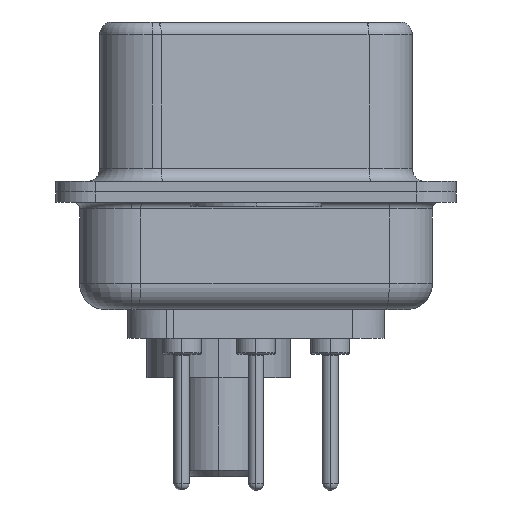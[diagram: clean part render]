
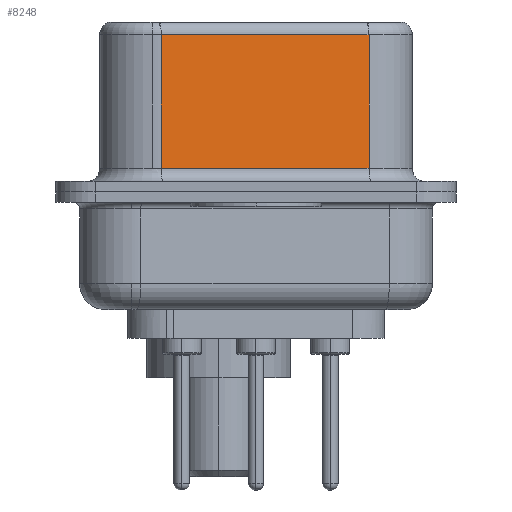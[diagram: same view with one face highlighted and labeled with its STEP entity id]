
A CAD part, left-side view. The second image highlights one B-rep face of the part: STEP entity #8248.
In plain terms, the highlighted planar face has unit normal (-0.985, -0.174, 0).
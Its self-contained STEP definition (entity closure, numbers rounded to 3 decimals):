
#238 = DIRECTION ( 'NONE',  ( 0.985, 0.174, 0. ) ) ;
#2399 = ORIENTED_EDGE ( 'NONE', *, *, #17463, .T. ) ;
#2860 = LINE ( 'NONE', #15412, #23816 ) ;
#3398 = CARTESIAN_POINT ( 'NONE',  ( 5.132, -4.322, 0.9 ) ) ;
#4527 = VERTEX_POINT ( 'NONE', #22207 ) ;
#5184 = VECTOR ( 'NONE', #6916, 1000. ) ;
#6916 = DIRECTION ( 'NONE',  ( 0., 0., -1. ) ) ;
#8248 = ADVANCED_FACE ( 'NONE', ( #8798 ), #12422, .F. ) ;
#8433 = CARTESIAN_POINT ( 'NONE',  ( 5.132, -4.322, 6.52 ) ) ;
#8798 = FACE_OUTER_BOUND ( 'NONE', #22012, .T. ) ;
#9192 = LINE ( 'NONE', #12974, #25461 ) ;
#9253 = VERTEX_POINT ( 'NONE', #9513 ) ;
#9513 = CARTESIAN_POINT ( 'NONE',  ( 3.73, 3.628, 0.9 ) ) ;
#10468 = LINE ( 'NONE', #14856, #5184 ) ;
#12422 = PLANE ( 'NONE',  #13414 ) ;
#12682 = VECTOR ( 'NONE', #23684, 1000. ) ;
#12974 = CARTESIAN_POINT ( 'NONE',  ( 5.132, -4.322, 6.02 ) ) ;
#13414 = AXIS2_PLACEMENT_3D ( 'NONE', #8433, #238, #14448 ) ;
#14448 = DIRECTION ( 'NONE',  ( -0.174, 0.985, 0. ) ) ;
#14601 = LINE ( 'NONE', #3398, #12682 ) ;
#14856 = CARTESIAN_POINT ( 'NONE',  ( 3.73, 3.628, 6.52 ) ) ;
#15024 = DIRECTION ( 'NONE',  ( -0.174, 0.985, 0. ) ) ;
#15412 = CARTESIAN_POINT ( 'NONE',  ( 5.132, -4.322, 6.52 ) ) ;
#17463 = EDGE_CURVE ( 'NONE', #9253, #25032, #14601, .T. ) ;
#17486 = DIRECTION ( 'NONE',  ( 0., 0., -1. ) ) ;
#19724 = EDGE_CURVE ( 'NONE', #23971, #25032, #2860, .T. ) ;
#20028 = ORIENTED_EDGE ( 'NONE', *, *, #20218, .T. ) ;
#20218 = EDGE_CURVE ( 'NONE', #23971, #4527, #9192, .T. ) ;
#22001 = ORIENTED_EDGE ( 'NONE', *, *, #19724, .F. ) ;
#22012 = EDGE_LOOP ( 'NONE', ( #22001, #20028, #23916, #2399 ) ) ;
#22207 = CARTESIAN_POINT ( 'NONE',  ( 3.73, 3.628, 6.02 ) ) ;
#22925 = CARTESIAN_POINT ( 'NONE',  ( 5.132, -4.322, 6.02 ) ) ;
#23388 = EDGE_CURVE ( 'NONE', #4527, #9253, #10468, .T. ) ;
#23684 = DIRECTION ( 'NONE',  ( 0.174, -0.985, 0. ) ) ;
#23816 = VECTOR ( 'NONE', #17486, 1000. ) ;
#23916 = ORIENTED_EDGE ( 'NONE', *, *, #23388, .T. ) ;
#23971 = VERTEX_POINT ( 'NONE', #22925 ) ;
#25011 = CARTESIAN_POINT ( 'NONE',  ( 5.132, -4.322, 0.9 ) ) ;
#25032 = VERTEX_POINT ( 'NONE', #25011 ) ;
#25461 = VECTOR ( 'NONE', #15024, 1000. ) ;
